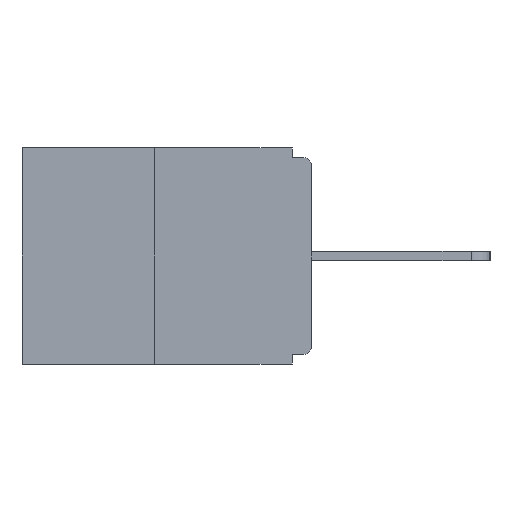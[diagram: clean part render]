
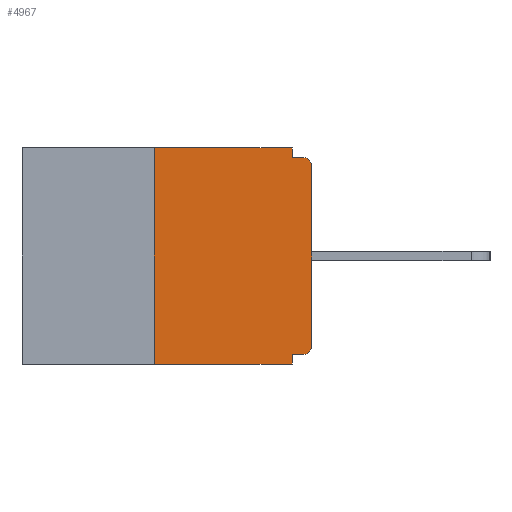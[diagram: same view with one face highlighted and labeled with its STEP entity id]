
A CAD part, left-side view. The second image highlights one B-rep face of the part: STEP entity #4967.
In plain terms, the highlighted planar face has unit normal (-1, 0, 0).
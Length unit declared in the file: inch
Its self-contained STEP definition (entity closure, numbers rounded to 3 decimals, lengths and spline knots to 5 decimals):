
#150 = EDGE_CURVE ( 'NONE', #10567, #7163, #9259, .T. ) ;
#398 = CARTESIAN_POINT ( 'NONE',  ( 0., 0.015, -0.313 ) ) ;
#548 = CARTESIAN_POINT ( 'NONE',  ( 0., 0.031, -0.343 ) ) ;
#555 = CARTESIAN_POINT ( 'NONE',  ( 0., 0.031, -0.343 ) ) ;
#820 = VECTOR ( 'NONE', #8642, 39.37008 ) ;
#1023 = CARTESIAN_POINT ( 'NONE',  ( 0., 0.031, 0. ) ) ;
#1550 = VERTEX_POINT ( 'NONE', #15761 ) ;
#1568 = CARTESIAN_POINT ( 'NONE',  ( 0., 0.015, -0.328 ) ) ;
#1858 = CARTESIAN_POINT ( 'NONE',  ( 0., 0.25, -0.343 ) ) ;
#1872 = VERTEX_POINT ( 'NONE', #1858 ) ;
#2335 = CARTESIAN_POINT ( 'NONE',  ( 0., 0.25, 0. ) ) ;
#2877 = EDGE_CURVE ( 'NONE', #1550, #8118, #16314, .T. ) ;
#2954 = ORIENTED_EDGE ( 'NONE', *, *, #7225, .F. ) ;
#3290 = CARTESIAN_POINT ( 'NONE',  ( 0., 0.031, -0.015 ) ) ;
#3503 = LINE ( 'NONE', #548, #11507 ) ;
#3988 = CARTESIAN_POINT ( 'NONE',  ( 0., 0.25, 0. ) ) ;
#4039 = DIRECTION ( 'NONE',  ( 1., 0., 0. ) ) ;
#4376 = DIRECTION ( 'NONE',  ( 0., 0., -1. ) ) ;
#4967 = ADVANCED_FACE ( 'NONE', ( #13272 ), #10227, .F. ) ;
#5038 = VECTOR ( 'NONE', #12501, 39.37008 ) ;
#5115 = DIRECTION ( 'NONE',  ( 0., 0., -1. ) ) ;
#5347 = CARTESIAN_POINT ( 'NONE',  ( 0., 0.46, -0.343 ) ) ;
#5489 = VERTEX_POINT ( 'NONE', #16596 ) ;
#5755 = CARTESIAN_POINT ( 'NONE',  ( 0., 0.46, 0. ) ) ;
#6004 = DIRECTION ( 'NONE',  ( -1., 0., 0. ) ) ;
#6131 = CIRCLE ( 'NONE', #12931, 0.015 ) ;
#6260 = DIRECTION ( 'NONE',  ( 0., 0., 1. ) ) ;
#6582 = DIRECTION ( 'NONE',  ( -1., 0., 0. ) ) ;
#6684 = LINE ( 'NONE', #1023, #17198 ) ;
#7015 = CARTESIAN_POINT ( 'NONE',  ( 0., 0.015, -0.015 ) ) ;
#7163 = VERTEX_POINT ( 'NONE', #11255 ) ;
#7225 = EDGE_CURVE ( 'NONE', #5489, #16011, #6684, .T. ) ;
#8108 = ORIENTED_EDGE ( 'NONE', *, *, #13027, .T. ) ;
#8118 = VERTEX_POINT ( 'NONE', #7015 ) ;
#8312 = EDGE_CURVE ( 'NONE', #16011, #8118, #12391, .T. ) ;
#8606 = VERTEX_POINT ( 'NONE', #13703 ) ;
#8624 = CARTESIAN_POINT ( 'NONE',  ( 0., 0.46, 0. ) ) ;
#8642 = DIRECTION ( 'NONE',  ( 0., 0., 1. ) ) ;
#8838 = DIRECTION ( 'NONE',  ( 0., -1., 0. ) ) ;
#9050 = VECTOR ( 'NONE', #11758, 39.37008 ) ;
#9056 = CARTESIAN_POINT ( 'NONE',  ( 0., 0.015, -0.03 ) ) ;
#9259 = LINE ( 'NONE', #15634, #5038 ) ;
#9342 = DIRECTION ( 'NONE',  ( 0., -1., 0. ) ) ;
#9699 = EDGE_CURVE ( 'NONE', #19233, #5489, #16552, .T. ) ;
#9837 = AXIS2_PLACEMENT_3D ( 'NONE', #9056, #6004, #4376 ) ;
#10004 = ORIENTED_EDGE ( 'NONE', *, *, #150, .F. ) ;
#10026 = VECTOR ( 'NONE', #6260, 39.37008 ) ;
#10227 = PLANE ( 'NONE',  #16823 ) ;
#10567 = VERTEX_POINT ( 'NONE', #1568 ) ;
#10741 = ORIENTED_EDGE ( 'NONE', *, *, #9699, .F. ) ;
#10788 = ORIENTED_EDGE ( 'NONE', *, *, #14489, .T. ) ;
#11084 = EDGE_CURVE ( 'NONE', #1872, #19233, #17880, .T. ) ;
#11255 = CARTESIAN_POINT ( 'NONE',  ( 0., 0.031, -0.328 ) ) ;
#11507 = VECTOR ( 'NONE', #5115, 39.37008 ) ;
#11622 = ORIENTED_EDGE ( 'NONE', *, *, #15737, .F. ) ;
#11758 = DIRECTION ( 'NONE',  ( 0., -1., 0. ) ) ;
#12194 = VERTEX_POINT ( 'NONE', #555 ) ;
#12248 = CARTESIAN_POINT ( 'NONE',  ( 0., 0., 0. ) ) ;
#12391 = LINE ( 'NONE', #18571, #17759 ) ;
#12446 = LINE ( 'NONE', #12248, #10026 ) ;
#12501 = DIRECTION ( 'NONE',  ( 0., 1., 0. ) ) ;
#12663 = ORIENTED_EDGE ( 'NONE', *, *, #2877, .T. ) ;
#12868 = DIRECTION ( 'NONE',  ( 0., 0., -1. ) ) ;
#12931 = AXIS2_PLACEMENT_3D ( 'NONE', #398, #6582, #12868 ) ;
#13027 = EDGE_CURVE ( 'NONE', #10567, #8606, #6131, .T. ) ;
#13064 = EDGE_CURVE ( 'NONE', #1872, #12194, #16320, .T. ) ;
#13272 = FACE_OUTER_BOUND ( 'NONE', #19517, .T. ) ;
#13703 = CARTESIAN_POINT ( 'NONE',  ( 0., 0., -0.313 ) ) ;
#14400 = VECTOR ( 'NONE', #8838, 39.37008 ) ;
#14489 = EDGE_CURVE ( 'NONE', #8606, #1550, #12446, .T. ) ;
#14567 = ORIENTED_EDGE ( 'NONE', *, *, #8312, .F. ) ;
#15249 = ORIENTED_EDGE ( 'NONE', *, *, #13064, .T. ) ;
#15634 = CARTESIAN_POINT ( 'NONE',  ( 0., 0., -0.328 ) ) ;
#15737 = EDGE_CURVE ( 'NONE', #7163, #12194, #3503, .T. ) ;
#15761 = CARTESIAN_POINT ( 'NONE',  ( 0., 0., -0.03 ) ) ;
#16011 = VERTEX_POINT ( 'NONE', #3290 ) ;
#16314 = CIRCLE ( 'NONE', #9837, 0.015 ) ;
#16320 = LINE ( 'NONE', #5347, #9050 ) ;
#16417 = DIRECTION ( 'NONE',  ( 0., 0., -1. ) ) ;
#16552 = LINE ( 'NONE', #8624, #14400 ) ;
#16596 = CARTESIAN_POINT ( 'NONE',  ( 0., 0.031, 0. ) ) ;
#16823 = AXIS2_PLACEMENT_3D ( 'NONE', #5755, #4039, #16417 ) ;
#17198 = VECTOR ( 'NONE', #19476, 39.37008 ) ;
#17263 = ORIENTED_EDGE ( 'NONE', *, *, #11084, .F. ) ;
#17759 = VECTOR ( 'NONE', #9342, 39.37008 ) ;
#17880 = LINE ( 'NONE', #3988, #820 ) ;
#18571 = CARTESIAN_POINT ( 'NONE',  ( 0., 0., -0.015 ) ) ;
#19233 = VERTEX_POINT ( 'NONE', #2335 ) ;
#19476 = DIRECTION ( 'NONE',  ( 0., 0., -1. ) ) ;
#19517 = EDGE_LOOP ( 'NONE', ( #10741, #17263, #15249, #11622, #10004, #8108, #10788, #12663, #14567, #2954 ) ) ;
